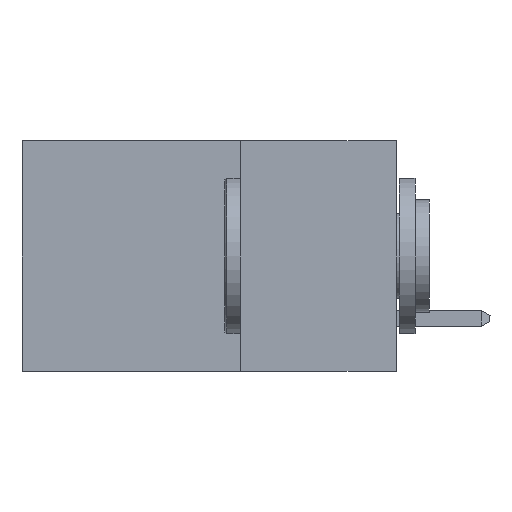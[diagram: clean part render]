
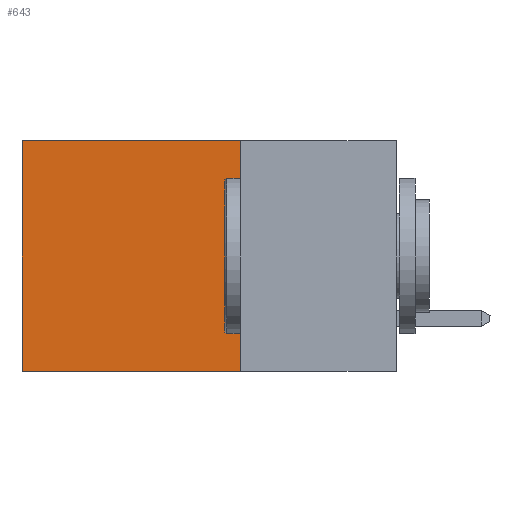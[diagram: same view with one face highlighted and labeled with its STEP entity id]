
A CAD part, left-side view. The second image highlights one B-rep face of the part: STEP entity #643.
In plain terms, the highlighted planar face has unit normal (-1, 0, 0).
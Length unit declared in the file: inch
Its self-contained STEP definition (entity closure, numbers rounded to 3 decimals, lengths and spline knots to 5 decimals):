
#563 = LINE ( 'NONE', #14417, #13077 ) ;
#643 = ADVANCED_FACE ( 'NONE', ( #11592 ), #9664, .F. ) ;
#654 = LINE ( 'NONE', #3014, #12621 ) ;
#1167 = ORIENTED_EDGE ( 'NONE', *, *, #15373, .T. ) ;
#1369 = VERTEX_POINT ( 'NONE', #15711 ) ;
#1837 = CARTESIAN_POINT ( 'NONE',  ( 0.2615, 0.6, 0. ) ) ;
#1971 = VECTOR ( 'NONE', #9832, 39.37008 ) ;
#2461 = VERTEX_POINT ( 'NONE', #1837 ) ;
#2822 = LINE ( 'NONE', #19640, #10994 ) ;
#3014 = CARTESIAN_POINT ( 'NONE',  ( 0.2615, 0.25, -0.37 ) ) ;
#4515 = VERTEX_POINT ( 'NONE', #16460 ) ;
#4731 = VERTEX_POINT ( 'NONE', #5404 ) ;
#5404 = CARTESIAN_POINT ( 'NONE',  ( 0.2615, 0.25, -0.37 ) ) ;
#5746 = EDGE_CURVE ( 'NONE', #4731, #4515, #654, .T. ) ;
#6834 = LINE ( 'NONE', #16377, #1971 ) ;
#6902 = DIRECTION ( 'NONE',  ( 0., 0., -1. ) ) ;
#7037 = AXIS2_PLACEMENT_3D ( 'NONE', #13678, #11782, #6902 ) ;
#7400 = ORIENTED_EDGE ( 'NONE', *, *, #5746, .F. ) ;
#9664 = PLANE ( 'NONE',  #7037 ) ;
#9832 = DIRECTION ( 'NONE',  ( 0., 1., 0. ) ) ;
#9896 = DIRECTION ( 'NONE',  ( 0., 0., -1. ) ) ;
#10994 = VECTOR ( 'NONE', #9896, 39.37008 ) ;
#11592 = FACE_OUTER_BOUND ( 'NONE', #17802, .T. ) ;
#11782 = DIRECTION ( 'NONE',  ( 1., 0., 0. ) ) ;
#12621 = VECTOR ( 'NONE', #16120, 39.37008 ) ;
#13077 = VECTOR ( 'NONE', #16069, 39.37008 ) ;
#13556 = EDGE_CURVE ( 'NONE', #1369, #4731, #2822, .T. ) ;
#13678 = CARTESIAN_POINT ( 'NONE',  ( 0.2615, 0.25, -0.37 ) ) ;
#14417 = CARTESIAN_POINT ( 'NONE',  ( 0.2615, 0.6, -0.37 ) ) ;
#15373 = EDGE_CURVE ( 'NONE', #1369, #2461, #6834, .T. ) ;
#15711 = CARTESIAN_POINT ( 'NONE',  ( 0.2615, 0.25, 0. ) ) ;
#16069 = DIRECTION ( 'NONE',  ( 0., 0., -1. ) ) ;
#16120 = DIRECTION ( 'NONE',  ( 0., 1., 0. ) ) ;
#16377 = CARTESIAN_POINT ( 'NONE',  ( 0.2615, 0.25, 0. ) ) ;
#16460 = CARTESIAN_POINT ( 'NONE',  ( 0.2615, 0.6, -0.37 ) ) ;
#17802 = EDGE_LOOP ( 'NONE', ( #21024, #7400, #19691, #1167 ) ) ;
#18616 = EDGE_CURVE ( 'NONE', #2461, #4515, #563, .T. ) ;
#19640 = CARTESIAN_POINT ( 'NONE',  ( 0.2615, 0.25, -0.37 ) ) ;
#19691 = ORIENTED_EDGE ( 'NONE', *, *, #13556, .F. ) ;
#21024 = ORIENTED_EDGE ( 'NONE', *, *, #18616, .T. ) ;
